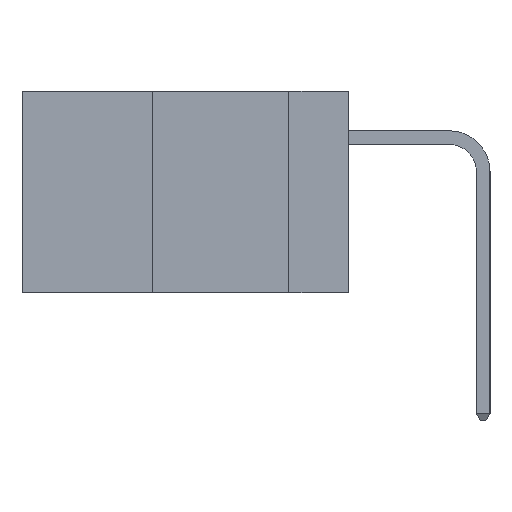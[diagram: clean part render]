
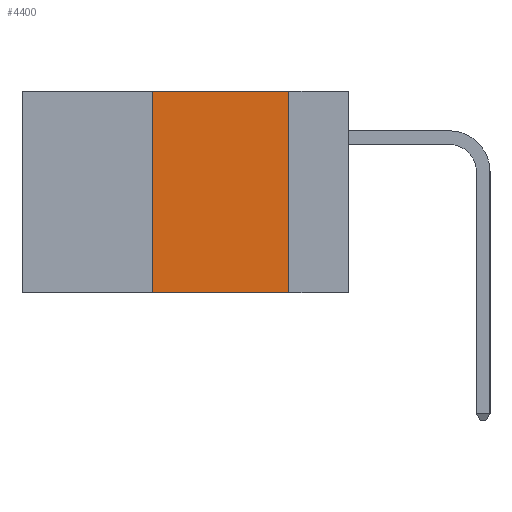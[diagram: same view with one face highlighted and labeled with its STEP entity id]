
A CAD part, left-side view. The second image highlights one B-rep face of the part: STEP entity #4400.
In plain terms, the highlighted planar face has unit normal (-1, 0, 0).
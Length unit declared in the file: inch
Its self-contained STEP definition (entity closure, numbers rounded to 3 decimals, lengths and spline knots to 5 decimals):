
#174 = ORIENTED_EDGE ( 'NONE', *, *, #621, .F. ) ;
#241 = VERTEX_POINT ( 'NONE', #1799 ) ;
#351 = DIRECTION ( 'NONE',  ( 0., 0., 1. ) ) ;
#457 = ORIENTED_EDGE ( 'NONE', *, *, #8530, .T. ) ;
#621 = EDGE_CURVE ( 'NONE', #241, #4350, #4369, .T. ) ;
#1322 = CARTESIAN_POINT ( 'NONE',  ( 0., 0.36, 0. ) ) ;
#1799 = CARTESIAN_POINT ( 'NONE',  ( 0., 0.36, 0. ) ) ;
#2008 = CARTESIAN_POINT ( 'NONE',  ( 0., 0.11, -0.37 ) ) ;
#2070 = VERTEX_POINT ( 'NONE', #2008 ) ;
#2380 = CARTESIAN_POINT ( 'NONE',  ( 0., 0.36, -0.37 ) ) ;
#2471 = DIRECTION ( 'NONE',  ( 0., 0., -1. ) ) ;
#2491 = EDGE_LOOP ( 'NONE', ( #8404, #174, #8658, #457 ) ) ;
#2492 = DIRECTION ( 'NONE',  ( 1., 0., 0. ) ) ;
#2503 = PLANE ( 'NONE',  #6050 ) ;
#2825 = CARTESIAN_POINT ( 'NONE',  ( 0., 0.6, 0. ) ) ;
#2833 = LINE ( 'NONE', #1322, #4763 ) ;
#4100 = VECTOR ( 'NONE', #5698, 39.37008 ) ;
#4218 = CARTESIAN_POINT ( 'NONE',  ( 0., 0.11, 0. ) ) ;
#4350 = VERTEX_POINT ( 'NONE', #4218 ) ;
#4369 = LINE ( 'NONE', #6320, #4100 ) ;
#4400 = ADVANCED_FACE ( 'NONE', ( #10079 ), #2503, .F. ) ;
#4757 = EDGE_CURVE ( 'NONE', #7588, #241, #2833, .T. ) ;
#4763 = VECTOR ( 'NONE', #351, 39.37008 ) ;
#5177 = CARTESIAN_POINT ( 'NONE',  ( 0., 0.11, 0. ) ) ;
#5698 = DIRECTION ( 'NONE',  ( 0., -1., 0. ) ) ;
#5934 = DIRECTION ( 'NONE',  ( 0., 0., -1. ) ) ;
#5948 = EDGE_CURVE ( 'NONE', #4350, #2070, #6152, .T. ) ;
#6050 = AXIS2_PLACEMENT_3D ( 'NONE', #2825, #2492, #2471 ) ;
#6152 = LINE ( 'NONE', #5177, #10157 ) ;
#6320 = CARTESIAN_POINT ( 'NONE',  ( 0., 0.6, 0. ) ) ;
#6346 = VECTOR ( 'NONE', #7266, 39.37008 ) ;
#6453 = CARTESIAN_POINT ( 'NONE',  ( 0., 0.6, -0.37 ) ) ;
#7266 = DIRECTION ( 'NONE',  ( 0., -1., 0. ) ) ;
#7588 = VERTEX_POINT ( 'NONE', #2380 ) ;
#7932 = LINE ( 'NONE', #6453, #6346 ) ;
#8404 = ORIENTED_EDGE ( 'NONE', *, *, #5948, .F. ) ;
#8530 = EDGE_CURVE ( 'NONE', #7588, #2070, #7932, .T. ) ;
#8658 = ORIENTED_EDGE ( 'NONE', *, *, #4757, .F. ) ;
#10079 = FACE_OUTER_BOUND ( 'NONE', #2491, .T. ) ;
#10157 = VECTOR ( 'NONE', #5934, 39.37008 ) ;
